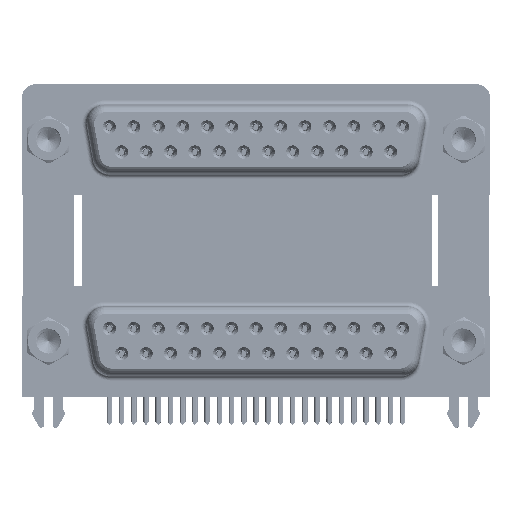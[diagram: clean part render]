
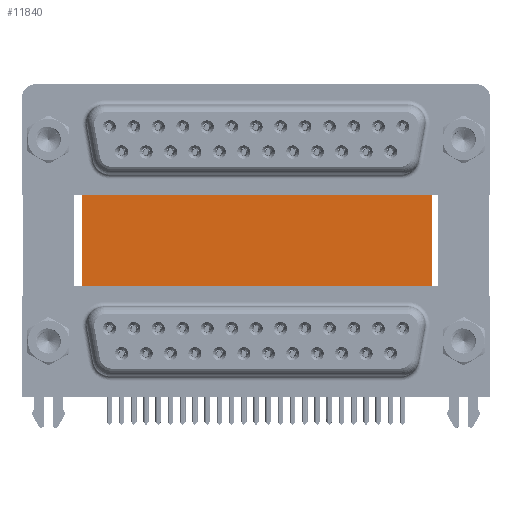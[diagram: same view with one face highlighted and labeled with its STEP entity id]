
A CAD part, top view. The second image highlights one B-rep face of the part: STEP entity #11840.
In plain terms, the highlighted planar face has unit normal (0, 0, 1).
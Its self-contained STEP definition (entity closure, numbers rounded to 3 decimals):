
#112 = VERTEX_POINT ( 'NONE', #975 ) ;
#975 = CARTESIAN_POINT ( 'NONE',  ( 43.43, -3.735, -12. ) ) ;
#4958 = DIRECTION ( 'NONE',  ( -1., 0., 0. ) ) ;
#5309 = LINE ( 'NONE', #62372, #6483 ) ;
#5591 = AXIS2_PLACEMENT_3D ( 'NONE', #52053, #31074, #4958 ) ;
#6483 = VECTOR ( 'NONE', #42428, 1000. ) ;
#8329 = CARTESIAN_POINT ( 'NONE',  ( 43.43, 16.585, -12. ) ) ;
#9022 = VERTEX_POINT ( 'NONE', #43279 ) ;
#10112 = PLANE ( 'NONE',  #5591 ) ;
#10398 = LINE ( 'NONE', #47181, #43961 ) ;
#11487 = EDGE_CURVE ( 'NONE', #9022, #18483, #10398, .T. ) ;
#11840 = ADVANCED_FACE ( 'NONE', ( #15250 ), #10112, .F. ) ;
#15250 = FACE_OUTER_BOUND ( 'NONE', #65262, .T. ) ;
#16313 = VECTOR ( 'NONE', #45098, 1000. ) ;
#18483 = VERTEX_POINT ( 'NONE', #8329 ) ;
#22723 = EDGE_CURVE ( 'NONE', #18483, #112, #60892, .T. ) ;
#28354 = ORIENTED_EDGE ( 'NONE', *, *, #66325, .T. ) ;
#31074 = DIRECTION ( 'NONE',  ( 0., 0., -1. ) ) ;
#34268 = CARTESIAN_POINT ( 'NONE',  ( 3.79, 16.585, -12. ) ) ;
#35557 = VERTEX_POINT ( 'NONE', #40587 ) ;
#35995 = EDGE_CURVE ( 'NONE', #9022, #35557, #39769, .T. ) ;
#36532 = ORIENTED_EDGE ( 'NONE', *, *, #22723, .F. ) ;
#39769 = LINE ( 'NONE', #34268, #60529 ) ;
#40587 = CARTESIAN_POINT ( 'NONE',  ( 3.79, -3.735, -12. ) ) ;
#42428 = DIRECTION ( 'NONE',  ( 1., 0., 0. ) ) ;
#43279 = CARTESIAN_POINT ( 'NONE',  ( 3.79, 16.585, -12. ) ) ;
#43961 = VECTOR ( 'NONE', #52329, 1000. ) ;
#45098 = DIRECTION ( 'NONE',  ( 0., -1., 0. ) ) ;
#47181 = CARTESIAN_POINT ( 'NONE',  ( 3.79, 16.585, -12. ) ) ;
#52053 = CARTESIAN_POINT ( 'NONE',  ( 3.79, 16.585, -12. ) ) ;
#52329 = DIRECTION ( 'NONE',  ( 1., 0., 0. ) ) ;
#53923 = ORIENTED_EDGE ( 'NONE', *, *, #11487, .F. ) ;
#55236 = DIRECTION ( 'NONE',  ( 0., -1., 0. ) ) ;
#60529 = VECTOR ( 'NONE', #55236, 1000. ) ;
#60892 = LINE ( 'NONE', #65358, #16313 ) ;
#62372 = CARTESIAN_POINT ( 'NONE',  ( 3.79, -3.735, -12. ) ) ;
#62741 = ORIENTED_EDGE ( 'NONE', *, *, #35995, .T. ) ;
#65262 = EDGE_LOOP ( 'NONE', ( #28354, #36532, #53923, #62741 ) ) ;
#65358 = CARTESIAN_POINT ( 'NONE',  ( 43.43, 16.585, -12. ) ) ;
#66325 = EDGE_CURVE ( 'NONE', #35557, #112, #5309, .T. ) ;
